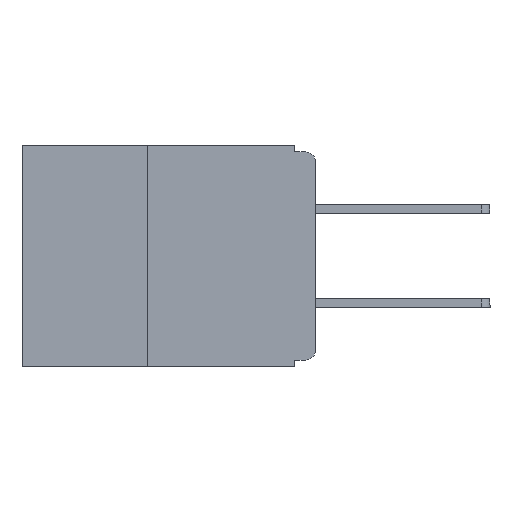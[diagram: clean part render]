
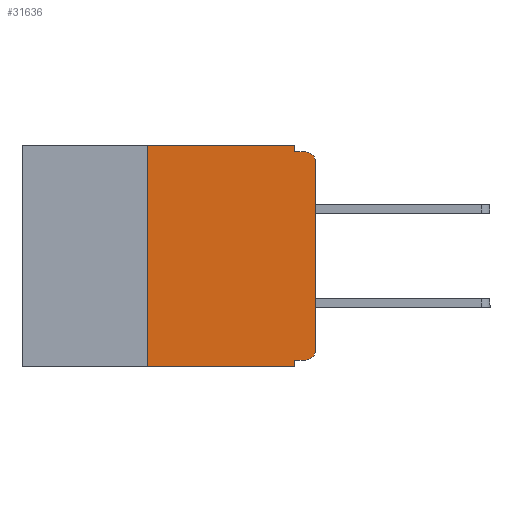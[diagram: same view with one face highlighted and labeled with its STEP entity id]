
A CAD part, left-side view. The second image highlights one B-rep face of the part: STEP entity #31636.
In plain terms, the highlighted planar face has unit normal (-1, 0, 0).
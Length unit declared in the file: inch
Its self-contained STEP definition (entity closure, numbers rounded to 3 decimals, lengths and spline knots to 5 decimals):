
#181 = CARTESIAN_POINT ( 'NONE',  ( 0., 0.031, 0. ) ) ;
#349 = CARTESIAN_POINT ( 'NONE',  ( 0., 0.031, -0.32 ) ) ;
#1483 = VERTEX_POINT ( 'NONE', #17245 ) ;
#1563 = DIRECTION ( 'NONE',  ( 0., -1., 0. ) ) ;
#1570 = DIRECTION ( 'NONE',  ( 1., 0., 0. ) ) ;
#1603 = CARTESIAN_POINT ( 'NONE',  ( 0., 0.437, -0.33 ) ) ;
#1709 = EDGE_CURVE ( 'NONE', #5395, #16134, #27035, .T. ) ;
#2093 = DIRECTION ( 'NONE',  ( -1., 0., 0. ) ) ;
#2770 = ORIENTED_EDGE ( 'NONE', *, *, #12241, .F. ) ;
#2896 = VERTEX_POINT ( 'NONE', #29015 ) ;
#2956 = LINE ( 'NONE', #24107, #30267 ) ;
#3250 = ORIENTED_EDGE ( 'NONE', *, *, #12490, .T. ) ;
#3901 = EDGE_CURVE ( 'NONE', #16134, #30260, #9979, .T. ) ;
#5395 = VERTEX_POINT ( 'NONE', #15807 ) ;
#6168 = LINE ( 'NONE', #27229, #33991 ) ;
#6213 = EDGE_CURVE ( 'NONE', #5395, #1483, #15450, .T. ) ;
#6928 = DIRECTION ( 'NONE',  ( 0., 0., -1. ) ) ;
#7860 = VERTEX_POINT ( 'NONE', #22927 ) ;
#8594 = CARTESIAN_POINT ( 'NONE',  ( 0., 0.015, -0.32 ) ) ;
#8794 = CARTESIAN_POINT ( 'NONE',  ( 0., 0.031, 0. ) ) ;
#9385 = DIRECTION ( 'NONE',  ( 0., -1., 0. ) ) ;
#9556 = CARTESIAN_POINT ( 'NONE',  ( 0., 0.437, 0. ) ) ;
#9811 = VECTOR ( 'NONE', #1563, 39.37008 ) ;
#9979 = LINE ( 'NONE', #9556, #23602 ) ;
#11361 = CARTESIAN_POINT ( 'NONE',  ( 0., 0.25, 0. ) ) ;
#12241 = EDGE_CURVE ( 'NONE', #30260, #2896, #12828, .T. ) ;
#12490 = EDGE_CURVE ( 'NONE', #25249, #19029, #18767, .T. ) ;
#12671 = VECTOR ( 'NONE', #25732, 39.37008 ) ;
#12828 = LINE ( 'NONE', #181, #26346 ) ;
#13229 = DIRECTION ( 'NONE',  ( 0., 0., 1. ) ) ;
#13383 = DIRECTION ( 'NONE',  ( -1., 0., 0. ) ) ;
#15176 = EDGE_CURVE ( 'NONE', #2896, #7860, #6168, .T. ) ;
#15450 = LINE ( 'NONE', #1603, #9811 ) ;
#15807 = CARTESIAN_POINT ( 'NONE',  ( 0., 0.25, -0.33 ) ) ;
#16134 = VERTEX_POINT ( 'NONE', #11361 ) ;
#16478 = CARTESIAN_POINT ( 'NONE',  ( 0., 0., -0.305 ) ) ;
#16576 = DIRECTION ( 'NONE',  ( 0., -1., 0. ) ) ;
#17153 = ORIENTED_EDGE ( 'NONE', *, *, #31231, .T. ) ;
#17203 = VECTOR ( 'NONE', #21384, 39.37008 ) ;
#17245 = CARTESIAN_POINT ( 'NONE',  ( 0., 0.031, -0.33 ) ) ;
#17298 = VERTEX_POINT ( 'NONE', #349 ) ;
#17441 = CARTESIAN_POINT ( 'NONE',  ( 0., 0., -0.025 ) ) ;
#18014 = ORIENTED_EDGE ( 'NONE', *, *, #6213, .T. ) ;
#18033 = VERTEX_POINT ( 'NONE', #17441 ) ;
#18207 = CARTESIAN_POINT ( 'NONE',  ( 0., 0.437, 0. ) ) ;
#18358 = EDGE_CURVE ( 'NONE', #18033, #7860, #26862, .T. ) ;
#18691 = CARTESIAN_POINT ( 'NONE',  ( 0., 0., -0.32 ) ) ;
#18713 = CARTESIAN_POINT ( 'NONE',  ( 0., 0.015, -0.305 ) ) ;
#18767 = CIRCLE ( 'NONE', #30477, 0.015 ) ;
#19029 = VERTEX_POINT ( 'NONE', #16478 ) ;
#19118 = AXIS2_PLACEMENT_3D ( 'NONE', #29461, #13383, #32070 ) ;
#19638 = ORIENTED_EDGE ( 'NONE', *, *, #15176, .F. ) ;
#20471 = EDGE_LOOP ( 'NONE', ( #17153, #25102, #19638, #2770, #34120, #20935, #18014, #28467, #33358, #3250 ) ) ;
#20696 = AXIS2_PLACEMENT_3D ( 'NONE', #18207, #1570, #20893 ) ;
#20786 = PLANE ( 'NONE',  #20696 ) ;
#20893 = DIRECTION ( 'NONE',  ( 0., 0., -1. ) ) ;
#20935 = ORIENTED_EDGE ( 'NONE', *, *, #1709, .F. ) ;
#21384 = DIRECTION ( 'NONE',  ( 0., 1., 0. ) ) ;
#21405 = DIRECTION ( 'NONE',  ( 0., 0., -1. ) ) ;
#22927 = CARTESIAN_POINT ( 'NONE',  ( 0., 0.015, -0.01 ) ) ;
#23602 = VECTOR ( 'NONE', #9385, 39.37008 ) ;
#23740 = FACE_OUTER_BOUND ( 'NONE', #20471, .T. ) ;
#24107 = CARTESIAN_POINT ( 'NONE',  ( 0., 0., 0. ) ) ;
#24181 = VECTOR ( 'NONE', #6928, 39.37008 ) ;
#24217 = EDGE_CURVE ( 'NONE', #17298, #1483, #24991, .T. ) ;
#24991 = LINE ( 'NONE', #33770, #24181 ) ;
#25102 = ORIENTED_EDGE ( 'NONE', *, *, #18358, .T. ) ;
#25249 = VERTEX_POINT ( 'NONE', #8594 ) ;
#25732 = DIRECTION ( 'NONE',  ( 0., 0., 1. ) ) ;
#26346 = VECTOR ( 'NONE', #30955, 39.37008 ) ;
#26862 = CIRCLE ( 'NONE', #19118, 0.015 ) ;
#27035 = LINE ( 'NONE', #30551, #12671 ) ;
#27229 = CARTESIAN_POINT ( 'NONE',  ( 0., 0., -0.01 ) ) ;
#28467 = ORIENTED_EDGE ( 'NONE', *, *, #24217, .F. ) ;
#29015 = CARTESIAN_POINT ( 'NONE',  ( 0., 0.031, -0.01 ) ) ;
#29461 = CARTESIAN_POINT ( 'NONE',  ( 0., 0.015, -0.025 ) ) ;
#30260 = VERTEX_POINT ( 'NONE', #8794 ) ;
#30267 = VECTOR ( 'NONE', #13229, 39.37008 ) ;
#30477 = AXIS2_PLACEMENT_3D ( 'NONE', #18713, #2093, #21405 ) ;
#30551 = CARTESIAN_POINT ( 'NONE',  ( 0., 0.25, -0.33 ) ) ;
#30955 = DIRECTION ( 'NONE',  ( 0., 0., -1. ) ) ;
#31231 = EDGE_CURVE ( 'NONE', #19029, #18033, #2956, .T. ) ;
#31343 = LINE ( 'NONE', #18691, #17203 ) ;
#31636 = ADVANCED_FACE ( 'NONE', ( #23740 ), #20786, .F. ) ;
#32070 = DIRECTION ( 'NONE',  ( 0., 0., -1. ) ) ;
#33358 = ORIENTED_EDGE ( 'NONE', *, *, #34798, .F. ) ;
#33770 = CARTESIAN_POINT ( 'NONE',  ( 0., 0.031, -0.33 ) ) ;
#33991 = VECTOR ( 'NONE', #16576, 39.37008 ) ;
#34120 = ORIENTED_EDGE ( 'NONE', *, *, #3901, .F. ) ;
#34798 = EDGE_CURVE ( 'NONE', #25249, #17298, #31343, .T. ) ;
